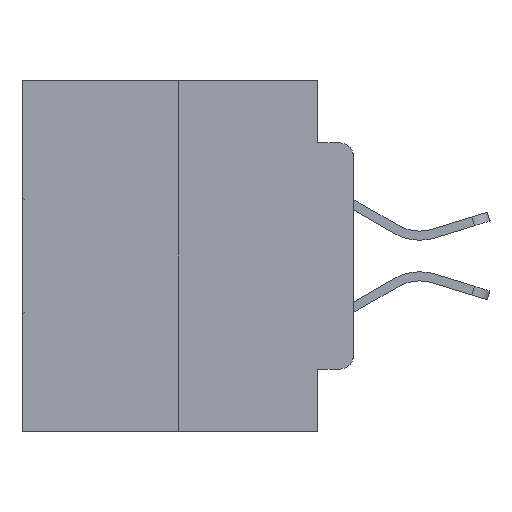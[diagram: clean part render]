
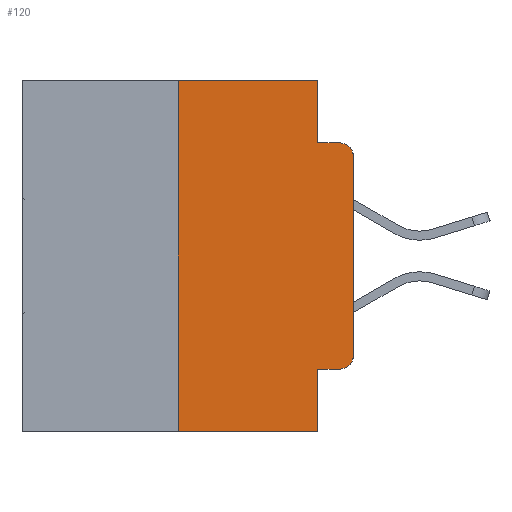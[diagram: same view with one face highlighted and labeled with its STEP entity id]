
A CAD part, left-side view. The second image highlights one B-rep face of the part: STEP entity #120.
In plain terms, the highlighted planar face has unit normal (-1, 0, 0).
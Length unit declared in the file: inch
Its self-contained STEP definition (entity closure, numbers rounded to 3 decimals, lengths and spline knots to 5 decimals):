
#120 = ADVANCED_FACE ( 'NONE', ( #9833 ), #17646, .F. ) ;
#800 = CARTESIAN_POINT ( 'NONE',  ( 0., 0.051, 0. ) ) ;
#1197 = EDGE_CURVE ( 'NONE', #22855, #21781, #15515, .T. ) ;
#1592 = VECTOR ( 'NONE', #18648, 39.37008 ) ;
#2473 = VECTOR ( 'NONE', #17365, 39.37008 ) ;
#2589 = VECTOR ( 'NONE', #19895, 39.37008 ) ;
#2827 = EDGE_CURVE ( 'NONE', #3424, #21781, #6245, .T. ) ;
#2831 = ORIENTED_EDGE ( 'NONE', *, *, #18224, .F. ) ;
#2938 = CARTESIAN_POINT ( 'NONE',  ( 0., 0.473, 0. ) ) ;
#3158 = CIRCLE ( 'NONE', #10768, 0.02 ) ;
#3399 = VERTEX_POINT ( 'NONE', #25424 ) ;
#3424 = VERTEX_POINT ( 'NONE', #23142 ) ;
#3555 = VERTEX_POINT ( 'NONE', #18833 ) ;
#4499 = EDGE_CURVE ( 'NONE', #9983, #3424, #14872, .T. ) ;
#5041 = CARTESIAN_POINT ( 'NONE',  ( 0., 0.473, -0.5 ) ) ;
#5449 = DIRECTION ( 'NONE',  ( 1., 0., 0. ) ) ;
#5819 = CARTESIAN_POINT ( 'NONE',  ( 0., 0.02, -0.3915 ) ) ;
#6045 = DIRECTION ( 'NONE',  ( 0., -1., 0. ) ) ;
#6245 = CIRCLE ( 'NONE', #9365, 0.02 ) ;
#6507 = CARTESIAN_POINT ( 'NONE',  ( 0., 0.25, 0. ) ) ;
#6585 = VECTOR ( 'NONE', #15482, 39.37008 ) ;
#7062 = VECTOR ( 'NONE', #28090, 39.37008 ) ;
#7523 = DIRECTION ( 'NONE',  ( 0., -1., 0. ) ) ;
#8239 = EDGE_CURVE ( 'NONE', #3555, #9271, #26008, .T. ) ;
#8308 = DIRECTION ( 'NONE',  ( 0., 0., -1. ) ) ;
#8644 = ORIENTED_EDGE ( 'NONE', *, *, #8239, .T. ) ;
#8751 = CARTESIAN_POINT ( 'NONE',  ( 0., 0.051, -0.5 ) ) ;
#9024 = VERTEX_POINT ( 'NONE', #22522 ) ;
#9271 = VERTEX_POINT ( 'NONE', #8751 ) ;
#9365 = AXIS2_PLACEMENT_3D ( 'NONE', #11343, #28113, #13769 ) ;
#9732 = VERTEX_POINT ( 'NONE', #24982 ) ;
#9833 = FACE_OUTER_BOUND ( 'NONE', #13476, .T. ) ;
#9983 = VERTEX_POINT ( 'NONE', #13814 ) ;
#10181 = ORIENTED_EDGE ( 'NONE', *, *, #13317, .T. ) ;
#10768 = AXIS2_PLACEMENT_3D ( 'NONE', #5819, #22813, #8308 ) ;
#11343 = CARTESIAN_POINT ( 'NONE',  ( 0., 0.02, -0.1085 ) ) ;
#11693 = EDGE_CURVE ( 'NONE', #15249, #9983, #3158, .T. ) ;
#13060 = LINE ( 'NONE', #25024, #6585 ) ;
#13317 = EDGE_CURVE ( 'NONE', #9024, #15249, #21069, .T. ) ;
#13476 = EDGE_LOOP ( 'NONE', ( #21156, #28184, #22634, #17024, #31172, #19291, #8644, #2831, #10181, #17417 ) ) ;
#13769 = DIRECTION ( 'NONE',  ( 0., 0., -1. ) ) ;
#13814 = CARTESIAN_POINT ( 'NONE',  ( 0., 0., -0.3915 ) ) ;
#14029 = LINE ( 'NONE', #800, #26791 ) ;
#14872 = LINE ( 'NONE', #17473, #2589 ) ;
#15249 = VERTEX_POINT ( 'NONE', #18856 ) ;
#15482 = DIRECTION ( 'NONE',  ( 0., 0., -1. ) ) ;
#15515 = LINE ( 'NONE', #17260, #2473 ) ;
#16285 = VECTOR ( 'NONE', #6045, 39.37008 ) ;
#17024 = ORIENTED_EDGE ( 'NONE', *, *, #21442, .F. ) ;
#17260 = CARTESIAN_POINT ( 'NONE',  ( 0., 0.051, -0.0885 ) ) ;
#17365 = DIRECTION ( 'NONE',  ( 0., -1., 0. ) ) ;
#17417 = ORIENTED_EDGE ( 'NONE', *, *, #11693, .T. ) ;
#17473 = CARTESIAN_POINT ( 'NONE',  ( 0., 0., 0. ) ) ;
#17646 = PLANE ( 'NONE',  #22894 ) ;
#17951 = DIRECTION ( 'NONE',  ( 0., 0., -1. ) ) ;
#18224 = EDGE_CURVE ( 'NONE', #9024, #9271, #14029, .T. ) ;
#18648 = DIRECTION ( 'NONE',  ( 0., -1., 0. ) ) ;
#18833 = CARTESIAN_POINT ( 'NONE',  ( 0., 0.25, -0.5 ) ) ;
#18856 = CARTESIAN_POINT ( 'NONE',  ( 0., 0.02, -0.4115 ) ) ;
#19291 = ORIENTED_EDGE ( 'NONE', *, *, #19831, .F. ) ;
#19831 = EDGE_CURVE ( 'NONE', #3555, #9732, #21501, .T. ) ;
#19895 = DIRECTION ( 'NONE',  ( 0., 0., 1. ) ) ;
#21069 = LINE ( 'NONE', #28093, #1592 ) ;
#21156 = ORIENTED_EDGE ( 'NONE', *, *, #4499, .T. ) ;
#21442 = EDGE_CURVE ( 'NONE', #3399, #22855, #13060, .T. ) ;
#21501 = LINE ( 'NONE', #6507, #7062 ) ;
#21781 = VERTEX_POINT ( 'NONE', #26250 ) ;
#22448 = DIRECTION ( 'NONE',  ( 0., 0., -1. ) ) ;
#22522 = CARTESIAN_POINT ( 'NONE',  ( 0., 0.051, -0.4115 ) ) ;
#22634 = ORIENTED_EDGE ( 'NONE', *, *, #1197, .F. ) ;
#22659 = LINE ( 'NONE', #25418, #16285 ) ;
#22813 = DIRECTION ( 'NONE',  ( -1., 0., 0. ) ) ;
#22855 = VERTEX_POINT ( 'NONE', #27288 ) ;
#22894 = AXIS2_PLACEMENT_3D ( 'NONE', #2938, #5449, #22448 ) ;
#23142 = CARTESIAN_POINT ( 'NONE',  ( 0., 0., -0.1085 ) ) ;
#24982 = CARTESIAN_POINT ( 'NONE',  ( 0., 0.25, 0. ) ) ;
#25024 = CARTESIAN_POINT ( 'NONE',  ( 0., 0.051, 0. ) ) ;
#25266 = VECTOR ( 'NONE', #7523, 39.37008 ) ;
#25418 = CARTESIAN_POINT ( 'NONE',  ( 0., 0.473, 0. ) ) ;
#25424 = CARTESIAN_POINT ( 'NONE',  ( 0., 0.051, 0. ) ) ;
#26008 = LINE ( 'NONE', #5041, #25266 ) ;
#26250 = CARTESIAN_POINT ( 'NONE',  ( 0., 0.02, -0.0885 ) ) ;
#26791 = VECTOR ( 'NONE', #17951, 39.37008 ) ;
#27288 = CARTESIAN_POINT ( 'NONE',  ( 0., 0.051, -0.0885 ) ) ;
#28090 = DIRECTION ( 'NONE',  ( 0., 0., 1. ) ) ;
#28093 = CARTESIAN_POINT ( 'NONE',  ( 0., 0.051, -0.4115 ) ) ;
#28113 = DIRECTION ( 'NONE',  ( -1., 0., 0. ) ) ;
#28184 = ORIENTED_EDGE ( 'NONE', *, *, #2827, .T. ) ;
#28987 = EDGE_CURVE ( 'NONE', #9732, #3399, #22659, .T. ) ;
#31172 = ORIENTED_EDGE ( 'NONE', *, *, #28987, .F. ) ;
